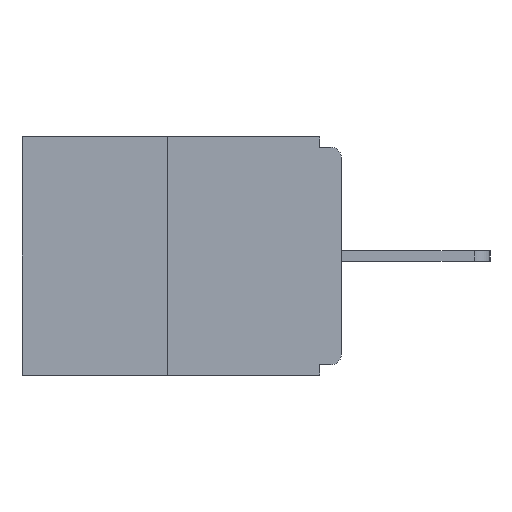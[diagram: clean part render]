
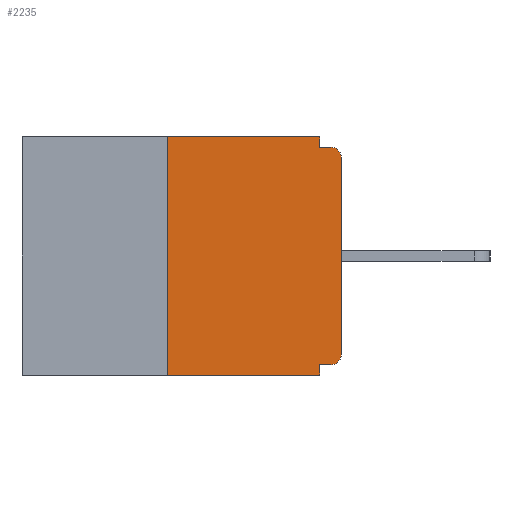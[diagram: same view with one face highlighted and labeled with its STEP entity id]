
A CAD part, left-side view. The second image highlights one B-rep face of the part: STEP entity #2235.
In plain terms, the highlighted planar face has unit normal (-1, 0, 0).
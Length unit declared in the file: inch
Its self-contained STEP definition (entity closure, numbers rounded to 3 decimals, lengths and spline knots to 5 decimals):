
#44 = CARTESIAN_POINT ( 'NONE',  ( 0., 0.015, -0.328 ) ) ;
#460 = DIRECTION ( 'NONE',  ( -1., 0., 0. ) ) ;
#464 = LINE ( 'NONE', #15747, #10512 ) ;
#630 = DIRECTION ( 'NONE',  ( -1., 0., 0. ) ) ;
#648 = CARTESIAN_POINT ( 'NONE',  ( 0., 0.25, -0.343 ) ) ;
#660 = CARTESIAN_POINT ( 'NONE',  ( 0., 0.015, -0.03 ) ) ;
#1275 = CARTESIAN_POINT ( 'NONE',  ( 0., 0., -0.328 ) ) ;
#1598 = CARTESIAN_POINT ( 'NONE',  ( 0., 0.25, 0. ) ) ;
#1701 = EDGE_CURVE ( 'NONE', #5800, #2879, #14506, .T. ) ;
#1852 = CARTESIAN_POINT ( 'NONE',  ( 0., 0., -0.03 ) ) ;
#2053 = CARTESIAN_POINT ( 'NONE',  ( 0., 0.031, 0. ) ) ;
#2235 = ADVANCED_FACE ( 'NONE', ( #8563 ), #5905, .F. ) ;
#2513 = EDGE_CURVE ( 'NONE', #3678, #2879, #10830, .T. ) ;
#2636 = ORIENTED_EDGE ( 'NONE', *, *, #2513, .T. ) ;
#2784 = CIRCLE ( 'NONE', #14123, 0.015 ) ;
#2879 = VERTEX_POINT ( 'NONE', #4398 ) ;
#3036 = ORIENTED_EDGE ( 'NONE', *, *, #10967, .T. ) ;
#3568 = VECTOR ( 'NONE', #17990, 39.37008 ) ;
#3617 = VERTEX_POINT ( 'NONE', #15353 ) ;
#3678 = VERTEX_POINT ( 'NONE', #1852 ) ;
#3797 = EDGE_CURVE ( 'NONE', #10955, #3617, #464, .T. ) ;
#3849 = EDGE_CURVE ( 'NONE', #11164, #5800, #9761, .T. ) ;
#4398 = CARTESIAN_POINT ( 'NONE',  ( 0., 0.015, -0.015 ) ) ;
#4480 = CARTESIAN_POINT ( 'NONE',  ( 0., 0.031, 0. ) ) ;
#4616 = ORIENTED_EDGE ( 'NONE', *, *, #7469, .T. ) ;
#4846 = AXIS2_PLACEMENT_3D ( 'NONE', #660, #460, #11231 ) ;
#5087 = DIRECTION ( 'NONE',  ( 0., -1., 0. ) ) ;
#5248 = DIRECTION ( 'NONE',  ( 0., 0., 1. ) ) ;
#5723 = ORIENTED_EDGE ( 'NONE', *, *, #15248, .F. ) ;
#5800 = VERTEX_POINT ( 'NONE', #8947 ) ;
#5905 = PLANE ( 'NONE',  #7905 ) ;
#6101 = ORIENTED_EDGE ( 'NONE', *, *, #15560, .F. ) ;
#6257 = ORIENTED_EDGE ( 'NONE', *, *, #3797, .T. ) ;
#6666 = LINE ( 'NONE', #7956, #14781 ) ;
#7274 = ORIENTED_EDGE ( 'NONE', *, *, #3849, .F. ) ;
#7469 = EDGE_CURVE ( 'NONE', #9480, #9571, #2784, .T. ) ;
#7514 = DIRECTION ( 'NONE',  ( 0., 1., 0. ) ) ;
#7905 = AXIS2_PLACEMENT_3D ( 'NONE', #10152, #8476, #14487 ) ;
#7956 = CARTESIAN_POINT ( 'NONE',  ( 0., 0., 0. ) ) ;
#8040 = CARTESIAN_POINT ( 'NONE',  ( 0., 0.015, -0.313 ) ) ;
#8264 = DIRECTION ( 'NONE',  ( 0., 0., -1. ) ) ;
#8399 = DIRECTION ( 'NONE',  ( 0., -1., 0. ) ) ;
#8476 = DIRECTION ( 'NONE',  ( 1., 0., 0. ) ) ;
#8563 = FACE_OUTER_BOUND ( 'NONE', #15679, .T. ) ;
#8947 = CARTESIAN_POINT ( 'NONE',  ( 0., 0.031, -0.015 ) ) ;
#9480 = VERTEX_POINT ( 'NONE', #44 ) ;
#9571 = VERTEX_POINT ( 'NONE', #12009 ) ;
#9761 = LINE ( 'NONE', #2053, #14582 ) ;
#10152 = CARTESIAN_POINT ( 'NONE',  ( 0., 0.46, 0. ) ) ;
#10512 = VECTOR ( 'NONE', #17313, 39.37008 ) ;
#10830 = CIRCLE ( 'NONE', #4846, 0.015 ) ;
#10955 = VERTEX_POINT ( 'NONE', #648 ) ;
#10967 = EDGE_CURVE ( 'NONE', #9571, #3678, #6666, .T. ) ;
#11164 = VERTEX_POINT ( 'NONE', #4480 ) ;
#11198 = VERTEX_POINT ( 'NONE', #1598 ) ;
#11231 = DIRECTION ( 'NONE',  ( 0., 0., -1. ) ) ;
#11981 = ORIENTED_EDGE ( 'NONE', *, *, #1701, .F. ) ;
#12009 = CARTESIAN_POINT ( 'NONE',  ( 0., 0., -0.313 ) ) ;
#12206 = VECTOR ( 'NONE', #5087, 39.37008 ) ;
#12992 = VERTEX_POINT ( 'NONE', #14545 ) ;
#13380 = LINE ( 'NONE', #19353, #3568 ) ;
#14123 = AXIS2_PLACEMENT_3D ( 'NONE', #8040, #630, #15513 ) ;
#14301 = CARTESIAN_POINT ( 'NONE',  ( 0., 0.25, 0. ) ) ;
#14371 = EDGE_CURVE ( 'NONE', #12992, #3617, #13380, .T. ) ;
#14396 = LINE ( 'NONE', #14301, #16454 ) ;
#14487 = DIRECTION ( 'NONE',  ( 0., 0., -1. ) ) ;
#14506 = LINE ( 'NONE', #17449, #17491 ) ;
#14545 = CARTESIAN_POINT ( 'NONE',  ( 0., 0.031, -0.328 ) ) ;
#14582 = VECTOR ( 'NONE', #8264, 39.37008 ) ;
#14781 = VECTOR ( 'NONE', #18481, 39.37008 ) ;
#15248 = EDGE_CURVE ( 'NONE', #9480, #12992, #16449, .T. ) ;
#15353 = CARTESIAN_POINT ( 'NONE',  ( 0., 0.031, -0.343 ) ) ;
#15513 = DIRECTION ( 'NONE',  ( 0., 0., -1. ) ) ;
#15560 = EDGE_CURVE ( 'NONE', #10955, #11198, #14396, .T. ) ;
#15679 = EDGE_LOOP ( 'NONE', ( #17094, #6101, #6257, #16365, #5723, #4616, #3036, #2636, #11981, #7274 ) ) ;
#15747 = CARTESIAN_POINT ( 'NONE',  ( 0., 0.46, -0.343 ) ) ;
#16365 = ORIENTED_EDGE ( 'NONE', *, *, #14371, .F. ) ;
#16449 = LINE ( 'NONE', #1275, #19293 ) ;
#16454 = VECTOR ( 'NONE', #5248, 39.37008 ) ;
#16989 = CARTESIAN_POINT ( 'NONE',  ( 0., 0.46, 0. ) ) ;
#17094 = ORIENTED_EDGE ( 'NONE', *, *, #18970, .F. ) ;
#17313 = DIRECTION ( 'NONE',  ( 0., -1., 0. ) ) ;
#17449 = CARTESIAN_POINT ( 'NONE',  ( 0., 0., -0.015 ) ) ;
#17491 = VECTOR ( 'NONE', #8399, 39.37008 ) ;
#17990 = DIRECTION ( 'NONE',  ( 0., 0., -1. ) ) ;
#18481 = DIRECTION ( 'NONE',  ( 0., 0., 1. ) ) ;
#18759 = LINE ( 'NONE', #16989, #12206 ) ;
#18970 = EDGE_CURVE ( 'NONE', #11198, #11164, #18759, .T. ) ;
#19293 = VECTOR ( 'NONE', #7514, 39.37008 ) ;
#19353 = CARTESIAN_POINT ( 'NONE',  ( 0., 0.031, -0.343 ) ) ;
